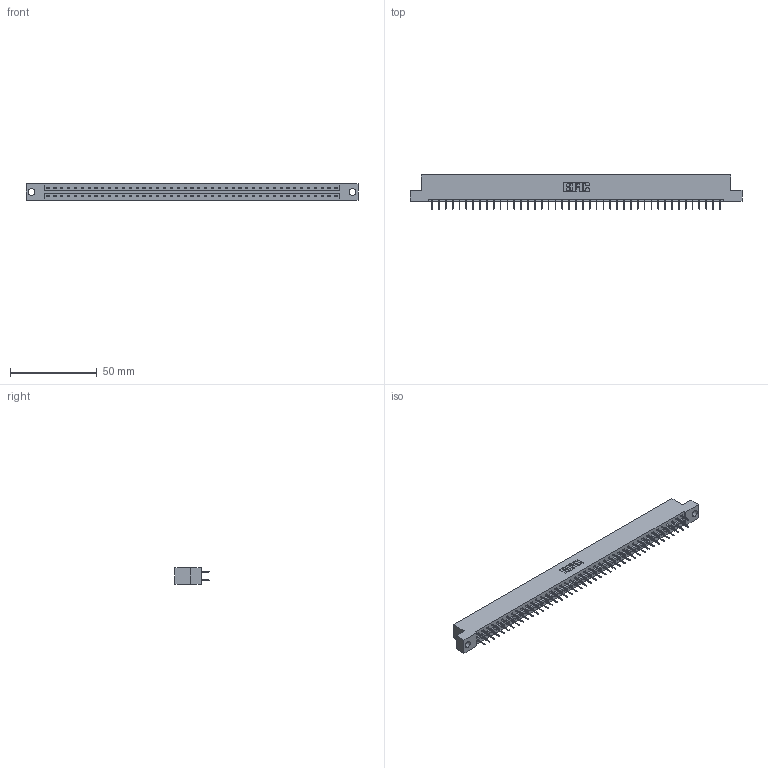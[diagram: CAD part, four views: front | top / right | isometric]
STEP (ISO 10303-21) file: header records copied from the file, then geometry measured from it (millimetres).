
FILE_DESCRIPTION (( 'STEP AP203' ), '1' );
FILE_NAME ('333-086-524-204.STEP', '2018-08-05T05:59:57', ( '' ), ( '' ), 'SwSTEP 2.0', 'SolidWorks 2016', '' );
FILE_SCHEMA (( 'CONFIG_CONTROL_DESIGN' ));
Length unit declared in the file: inch
Products named in the file (3): 345-292-001_345-293-124; 333-086-524-204; 333 Part_Flush - .156 Dia - TH
Assembly tree (87 placements, depth 2):
  333-086-524-204
    333 Part_Flush - .156 Dia - TH
    345-292-001_345-293-124  x86
Bounding box: 191.92 x 19.69 x 9.4 mm (x, y, z)
Volume: 19385.5 mm3; surface area: 22338.1 mm2
Topology: 87 solids, 87 shells, 4930 faces, 13985 edges, 8978 vertices
Faces by surface type: plane 3682, cylinder 1248
Entity records: 27611 total; most frequent: CARTESIAN_POINT 4574, ORIENTED_EDGE 4510, DIRECTION 3907, EDGE_CURVE 2255, LINE 2131, VECTOR 2131, VERTEX_POINT 1498, AXIS2_PLACEMENT_3D 888
